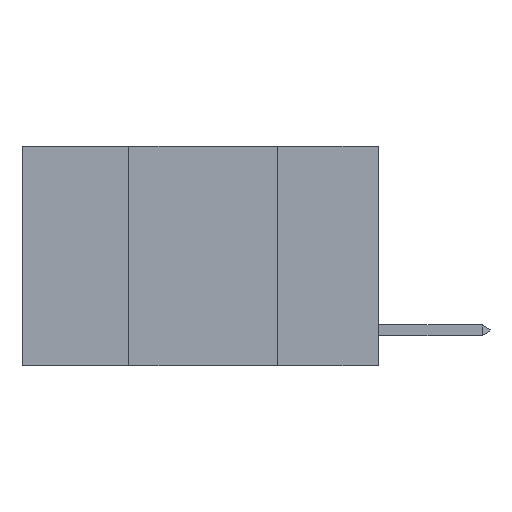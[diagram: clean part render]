
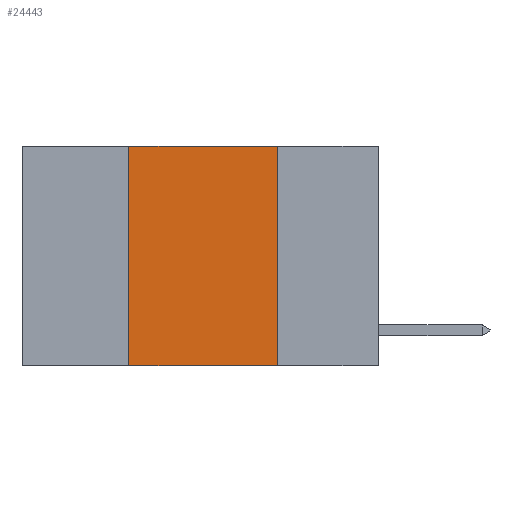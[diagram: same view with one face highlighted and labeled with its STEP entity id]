
A CAD part, left-side view. The second image highlights one B-rep face of the part: STEP entity #24443.
In plain terms, the highlighted planar face has unit normal (-1, 0, 0).
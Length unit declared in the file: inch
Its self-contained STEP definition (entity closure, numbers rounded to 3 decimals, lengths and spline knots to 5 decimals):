
#172 = LINE ( 'NONE', #25957, #17062 ) ;
#690 = DIRECTION ( 'NONE',  ( 0., -1., 0. ) ) ;
#2179 = CARTESIAN_POINT ( 'NONE',  ( 0., 0.17, 0. ) ) ;
#2503 = ORIENTED_EDGE ( 'NONE', *, *, #24037, .T. ) ;
#5155 = VERTEX_POINT ( 'NONE', #12811 ) ;
#5313 = VECTOR ( 'NONE', #10999, 39.37008 ) ;
#6192 = ORIENTED_EDGE ( 'NONE', *, *, #12885, .F. ) ;
#6249 = CARTESIAN_POINT ( 'NONE',  ( 0., 0.6, 0. ) ) ;
#6347 = DIRECTION ( 'NONE',  ( 0., 0., -1. ) ) ;
#7039 = EDGE_CURVE ( 'NONE', #22786, #28413, #17540, .T. ) ;
#8724 = CARTESIAN_POINT ( 'NONE',  ( 0., 0.6, -0.37 ) ) ;
#10779 = VERTEX_POINT ( 'NONE', #14463 ) ;
#10999 = DIRECTION ( 'NONE',  ( 0., 0., 1. ) ) ;
#12723 = AXIS2_PLACEMENT_3D ( 'NONE', #6249, #20124, #6347 ) ;
#12811 = CARTESIAN_POINT ( 'NONE',  ( 0., 0.17, 0. ) ) ;
#12885 = EDGE_CURVE ( 'NONE', #28413, #5155, #172, .T. ) ;
#13349 = DIRECTION ( 'NONE',  ( 0., -1., 0. ) ) ;
#13618 = DIRECTION ( 'NONE',  ( 0., 0., -1. ) ) ;
#14463 = CARTESIAN_POINT ( 'NONE',  ( 0., 0.17, -0.37 ) ) ;
#15357 = EDGE_LOOP ( 'NONE', ( #20562, #6192, #19132, #2503 ) ) ;
#15496 = VECTOR ( 'NONE', #13349, 39.37008 ) ;
#15931 = VECTOR ( 'NONE', #13618, 39.37008 ) ;
#17062 = VECTOR ( 'NONE', #690, 39.37008 ) ;
#17540 = LINE ( 'NONE', #24936, #5313 ) ;
#17791 = FACE_OUTER_BOUND ( 'NONE', #15357, .T. ) ;
#17809 = PLANE ( 'NONE',  #12723 ) ;
#19132 = ORIENTED_EDGE ( 'NONE', *, *, #7039, .F. ) ;
#20124 = DIRECTION ( 'NONE',  ( 1., 0., 0. ) ) ;
#20562 = ORIENTED_EDGE ( 'NONE', *, *, #22873, .F. ) ;
#21665 = LINE ( 'NONE', #8724, #15496 ) ;
#22786 = VERTEX_POINT ( 'NONE', #23474 ) ;
#22873 = EDGE_CURVE ( 'NONE', #5155, #10779, #28844, .T. ) ;
#23474 = CARTESIAN_POINT ( 'NONE',  ( 0., 0.42, -0.37 ) ) ;
#24037 = EDGE_CURVE ( 'NONE', #22786, #10779, #21665, .T. ) ;
#24443 = ADVANCED_FACE ( 'NONE', ( #17791 ), #17809, .F. ) ;
#24936 = CARTESIAN_POINT ( 'NONE',  ( 0., 0.42, 0. ) ) ;
#25957 = CARTESIAN_POINT ( 'NONE',  ( 0., 0.6, 0. ) ) ;
#28413 = VERTEX_POINT ( 'NONE', #29431 ) ;
#28844 = LINE ( 'NONE', #2179, #15931 ) ;
#29431 = CARTESIAN_POINT ( 'NONE',  ( 0., 0.42, 0. ) ) ;
